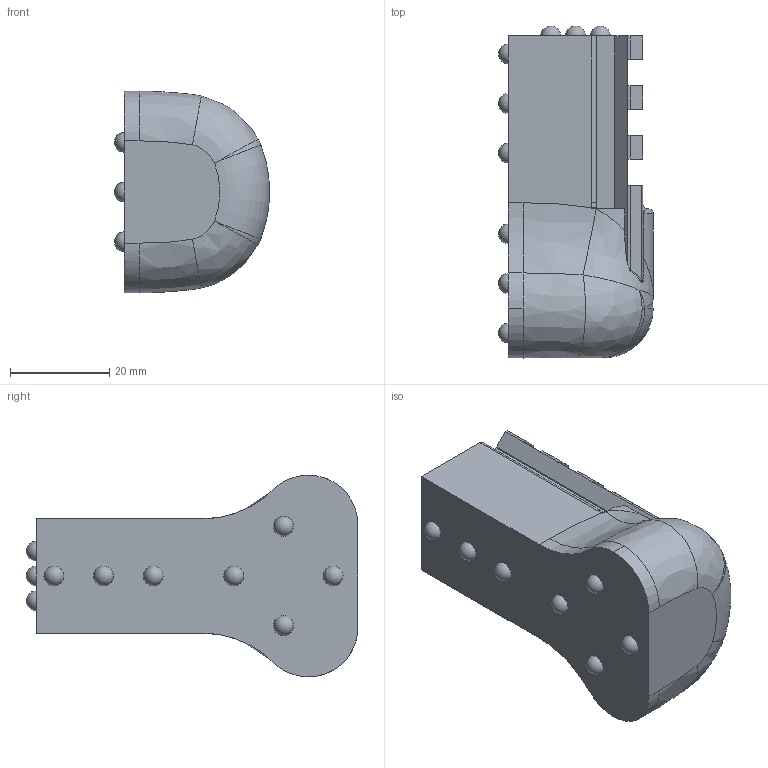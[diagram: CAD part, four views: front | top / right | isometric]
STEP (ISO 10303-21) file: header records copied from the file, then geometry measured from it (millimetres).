
FILE_DESCRIPTION (( 'STEP AP214' ), '1' );
FILE_NAME ('Stock Rail Rear.STEP', '2013-06-24T22:48:04', ( 'Asher' ), ( '' ), 'SwSTEP 2.0', 'SolidWorks 2013', '' );
FILE_SCHEMA (( 'AUTOMOTIVE_DESIGN' ));
Length unit declared in the file: millimetre
Products named in the file (1): Stock Rail Rear
Bounding box: 31.21 x 66.8 x 40.59 mm (x, y, z)
Volume: 43734.5 mm3; surface area: 8780 mm2
Topology: 1 solids, 1 shells, 95 faces, 267 edges, 161 vertices
Faces by surface type: plane 39, bspline 24, cylinder 19, sphere 11, torus 2
Entity records: 6326 total; most frequent: CARTESIAN_POINT 4164, ORIENTED_EDGE 478, DIRECTION 379, EDGE_CURVE 239, VERTEX_POINT 157, AXIS2_PLACEMENT_3D 130, VECTOR 119, LINE 119
